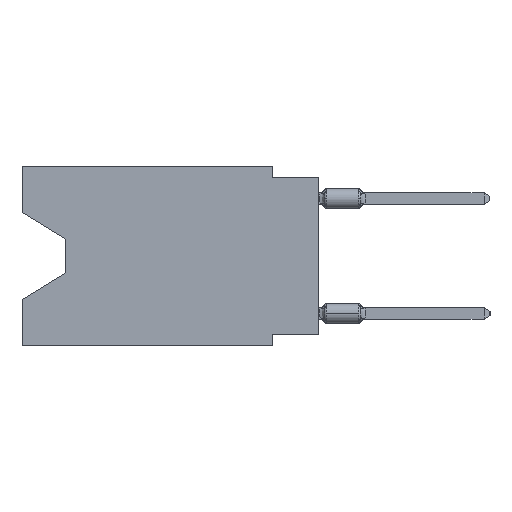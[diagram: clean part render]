
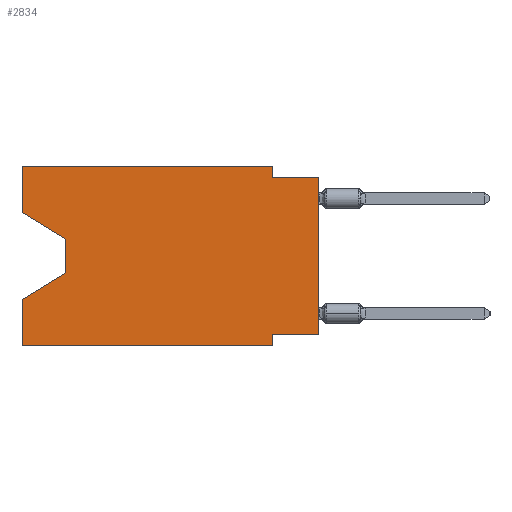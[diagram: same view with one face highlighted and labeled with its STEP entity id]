
A CAD part, left-side view. The second image highlights one B-rep face of the part: STEP entity #2834.
In plain terms, the highlighted planar face has unit normal (-1, 0, 0).
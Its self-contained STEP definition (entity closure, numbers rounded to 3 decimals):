
#41 = EDGE_CURVE ( 'NONE', #14926, #3255, #587, .T. ) ;
#112 = DIRECTION ( 'NONE',  ( 0., -1., 0. ) ) ;
#404 = VERTEX_POINT ( 'NONE', #25917 ) ;
#587 = LINE ( 'NONE', #11266, #18647 ) ;
#948 = CARTESIAN_POINT ( 'NONE',  ( 0., 16.383, -9.906 ) ) ;
#983 = VERTEX_POINT ( 'NONE', #24240 ) ;
#1197 = PLANE ( 'NONE',  #20467 ) ;
#1403 = DIRECTION ( 'NONE',  ( 0., 0.855, -0.519 ) ) ;
#1765 = VERTEX_POINT ( 'NONE', #22133 ) ;
#2044 = LINE ( 'NONE', #18819, #19008 ) ;
#2834 = ADVANCED_FACE ( 'NONE', ( #7609 ), #1197, .F. ) ;
#3142 = DIRECTION ( 'NONE',  ( 0., -1., 0. ) ) ;
#3255 = VERTEX_POINT ( 'NONE', #23975 ) ;
#3351 = CARTESIAN_POINT ( 'NONE',  ( 0., 0., -9.271 ) ) ;
#3383 = LINE ( 'NONE', #26167, #15808 ) ;
#3597 = CARTESIAN_POINT ( 'NONE',  ( 0., 13.97, -5.893 ) ) ;
#3901 = EDGE_CURVE ( 'NONE', #18936, #12788, #25398, .T. ) ;
#4115 = CARTESIAN_POINT ( 'NONE',  ( 0., 2.54, 0. ) ) ;
#4461 = CARTESIAN_POINT ( 'NONE',  ( 0., 13.97, -5.893 ) ) ;
#4882 = CARTESIAN_POINT ( 'NONE',  ( 0., 2.54, -9.906 ) ) ;
#5008 = ORIENTED_EDGE ( 'NONE', *, *, #17020, .F. ) ;
#5095 = VECTOR ( 'NONE', #22954, 1000. ) ;
#5339 = EDGE_CURVE ( 'NONE', #25682, #11260, #2044, .T. ) ;
#5412 = CARTESIAN_POINT ( 'NONE',  ( 0., 13.97, -4.013 ) ) ;
#5563 = DIRECTION ( 'NONE',  ( 1., 0., 0. ) ) ;
#5987 = VECTOR ( 'NONE', #1403, 1000. ) ;
#6536 = ORIENTED_EDGE ( 'NONE', *, *, #7509, .F. ) ;
#6691 = CARTESIAN_POINT ( 'NONE',  ( 0., 16.383, -2.546 ) ) ;
#6753 = VERTEX_POINT ( 'NONE', #21091 ) ;
#7028 = VECTOR ( 'NONE', #25679, 1000. ) ;
#7470 = LINE ( 'NONE', #15790, #10666 ) ;
#7490 = LINE ( 'NONE', #948, #19919 ) ;
#7509 = EDGE_CURVE ( 'NONE', #11260, #1765, #17211, .T. ) ;
#7609 = FACE_OUTER_BOUND ( 'NONE', #24598, .T. ) ;
#7618 = DIRECTION ( 'NONE',  ( 0., 0., 1. ) ) ;
#8009 = VERTEX_POINT ( 'NONE', #3351 ) ;
#8460 = ORIENTED_EDGE ( 'NONE', *, *, #20738, .F. ) ;
#9535 = DIRECTION ( 'NONE',  ( 0., 0., -1. ) ) ;
#10220 = EDGE_CURVE ( 'NONE', #8009, #20750, #22352, .T. ) ;
#10666 = VECTOR ( 'NONE', #19753, 1000. ) ;
#11260 = VERTEX_POINT ( 'NONE', #21424 ) ;
#11266 = CARTESIAN_POINT ( 'NONE',  ( 0., 16.383, 0. ) ) ;
#11691 = ORIENTED_EDGE ( 'NONE', *, *, #12471, .T. ) ;
#12329 = DIRECTION ( 'NONE',  ( 0., 1., 0. ) ) ;
#12470 = CARTESIAN_POINT ( 'NONE',  ( 0., 0., -0.635 ) ) ;
#12471 = EDGE_CURVE ( 'NONE', #14926, #404, #7490, .T. ) ;
#12788 = VERTEX_POINT ( 'NONE', #4461 ) ;
#12845 = CARTESIAN_POINT ( 'NONE',  ( 0., 13.97, -4.013 ) ) ;
#13227 = VECTOR ( 'NONE', #16939, 1000. ) ;
#14018 = CARTESIAN_POINT ( 'NONE',  ( 0., 16.383, 0. ) ) ;
#14403 = ORIENTED_EDGE ( 'NONE', *, *, #3901, .T. ) ;
#14926 = VERTEX_POINT ( 'NONE', #26933 ) ;
#15215 = DIRECTION ( 'NONE',  ( 0., 0., 1. ) ) ;
#15524 = LINE ( 'NONE', #4882, #15993 ) ;
#15790 = CARTESIAN_POINT ( 'NONE',  ( 0., 16.383, 0. ) ) ;
#15808 = VECTOR ( 'NONE', #12329, 1000. ) ;
#15964 = EDGE_CURVE ( 'NONE', #12788, #3255, #26654, .T. ) ;
#15993 = VECTOR ( 'NONE', #25760, 1000. ) ;
#16939 = DIRECTION ( 'NONE',  ( 0., -0.855, -0.519 ) ) ;
#17020 = EDGE_CURVE ( 'NONE', #6753, #404, #15524, .T. ) ;
#17061 = ORIENTED_EDGE ( 'NONE', *, *, #41, .F. ) ;
#17211 = LINE ( 'NONE', #4115, #5095 ) ;
#17572 = ORIENTED_EDGE ( 'NONE', *, *, #15964, .T. ) ;
#18129 = ORIENTED_EDGE ( 'NONE', *, *, #24593, .F. ) ;
#18386 = CARTESIAN_POINT ( 'NONE',  ( 0., 0., 0. ) ) ;
#18647 = VECTOR ( 'NONE', #15215, 1000. ) ;
#18819 = CARTESIAN_POINT ( 'NONE',  ( 0., 16.383, 0. ) ) ;
#18936 = VERTEX_POINT ( 'NONE', #5412 ) ;
#19008 = VECTOR ( 'NONE', #112, 1000. ) ;
#19021 = EDGE_CURVE ( 'NONE', #1765, #20750, #19745, .T. ) ;
#19191 = ORIENTED_EDGE ( 'NONE', *, *, #5339, .F. ) ;
#19745 = LINE ( 'NONE', #26161, #26310 ) ;
#19753 = DIRECTION ( 'NONE',  ( 0., 0., 1. ) ) ;
#19919 = VECTOR ( 'NONE', #3142, 1000. ) ;
#19944 = ORIENTED_EDGE ( 'NONE', *, *, #21250, .T. ) ;
#20443 = VECTOR ( 'NONE', #7618, 1000. ) ;
#20467 = AXIS2_PLACEMENT_3D ( 'NONE', #14018, #5563, #9535 ) ;
#20579 = CARTESIAN_POINT ( 'NONE',  ( 0., 16.383, 0. ) ) ;
#20738 = EDGE_CURVE ( 'NONE', #8009, #6753, #3383, .T. ) ;
#20750 = VERTEX_POINT ( 'NONE', #12470 ) ;
#21091 = CARTESIAN_POINT ( 'NONE',  ( 0., 2.54, -9.271 ) ) ;
#21250 = EDGE_CURVE ( 'NONE', #983, #18936, #22952, .T. ) ;
#21424 = CARTESIAN_POINT ( 'NONE',  ( 0., 2.54, 0. ) ) ;
#22133 = CARTESIAN_POINT ( 'NONE',  ( 0., 2.54, -0.635 ) ) ;
#22331 = DIRECTION ( 'NONE',  ( 0., -1., 0. ) ) ;
#22352 = LINE ( 'NONE', #18386, #20443 ) ;
#22952 = LINE ( 'NONE', #6691, #13227 ) ;
#22954 = DIRECTION ( 'NONE',  ( 0., 0., -1. ) ) ;
#23808 = ORIENTED_EDGE ( 'NONE', *, *, #10220, .T. ) ;
#23975 = CARTESIAN_POINT ( 'NONE',  ( 0., 16.383, -7.36 ) ) ;
#24240 = CARTESIAN_POINT ( 'NONE',  ( 0., 16.383, -2.546 ) ) ;
#24364 = ORIENTED_EDGE ( 'NONE', *, *, #19021, .F. ) ;
#24593 = EDGE_CURVE ( 'NONE', #983, #25682, #7470, .T. ) ;
#24598 = EDGE_LOOP ( 'NONE', ( #19944, #14403, #17572, #17061, #11691, #5008, #8460, #23808, #24364, #6536, #19191, #18129 ) ) ;
#25398 = LINE ( 'NONE', #12845, #7028 ) ;
#25679 = DIRECTION ( 'NONE',  ( 0., 0., -1. ) ) ;
#25682 = VERTEX_POINT ( 'NONE', #20579 ) ;
#25760 = DIRECTION ( 'NONE',  ( 0., 0., -1. ) ) ;
#25917 = CARTESIAN_POINT ( 'NONE',  ( 0., 2.54, -9.906 ) ) ;
#26161 = CARTESIAN_POINT ( 'NONE',  ( 0., 0., -0.635 ) ) ;
#26167 = CARTESIAN_POINT ( 'NONE',  ( 0., 0., -9.271 ) ) ;
#26310 = VECTOR ( 'NONE', #22331, 1000. ) ;
#26654 = LINE ( 'NONE', #3597, #5987 ) ;
#26933 = CARTESIAN_POINT ( 'NONE',  ( 0., 16.383, -9.906 ) ) ;
